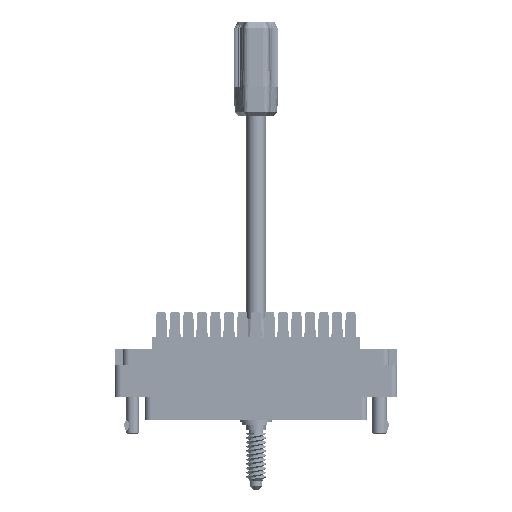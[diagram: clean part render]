
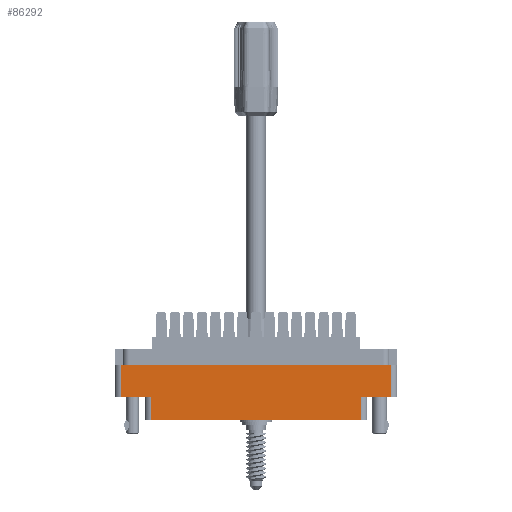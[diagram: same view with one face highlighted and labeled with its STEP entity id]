
A CAD part, front view. The second image highlights one B-rep face of the part: STEP entity #86292.
In plain terms, the highlighted planar face has unit normal (0, -1, 0).
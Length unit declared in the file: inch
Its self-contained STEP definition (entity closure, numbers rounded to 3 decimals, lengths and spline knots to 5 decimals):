
#207 = DIRECTION ( 'NONE',  ( 0., 0., 1. ) ) ;
#509 = ORIENTED_EDGE ( 'NONE', *, *, #36326, .T. ) ;
#2668 = DIRECTION ( 'NONE',  ( 0., 0., -1. ) ) ;
#3588 = LINE ( 'NONE', #40459, #69373 ) ;
#4038 = CARTESIAN_POINT ( 'NONE',  ( 1.297, -0.617, -0.274 ) ) ;
#4626 = LINE ( 'NONE', #34796, #83171 ) ;
#4710 = VECTOR ( 'NONE', #207, 39.37008 ) ;
#4845 = ORIENTED_EDGE ( 'NONE', *, *, #82349, .F. ) ;
#5252 = AXIS2_PLACEMENT_3D ( 'NONE', #71530, #87282, #94464 ) ;
#6112 = VECTOR ( 'NONE', #2668, 39.37008 ) ;
#8392 = DIRECTION ( 'NONE',  ( 1., 0., 0. ) ) ;
#12660 = ORIENTED_EDGE ( 'NONE', *, *, #57165, .T. ) ;
#14099 = PLANE ( 'NONE',  #5252 ) ;
#14154 = CARTESIAN_POINT ( 'NONE',  ( 0., -0.617, -0.578 ) ) ;
#14768 = VECTOR ( 'NONE', #71853, 39.37008 ) ;
#15088 = VECTOR ( 'NONE', #8392, 39.37008 ) ;
#15172 = EDGE_CURVE ( 'NONE', #60997, #40685, #4626, .T. ) ;
#16818 = ORIENTED_EDGE ( 'NONE', *, *, #30113, .T. ) ;
#22780 = VECTOR ( 'NONE', #74301, 39.37008 ) ;
#24410 = VERTEX_POINT ( 'NONE', #26943 ) ;
#26943 = CARTESIAN_POINT ( 'NONE',  ( 1.006, -0.617, -0.798 ) ) ;
#27652 = ORIENTED_EDGE ( 'NONE', *, *, #47729, .T. ) ;
#30113 = EDGE_CURVE ( 'NONE', #38169, #68191, #42983, .T. ) ;
#34769 = DIRECTION ( 'NONE',  ( -1., 0., 0. ) ) ;
#34796 = CARTESIAN_POINT ( 'NONE',  ( 0., -0.617, -0.274 ) ) ;
#36326 = EDGE_CURVE ( 'NONE', #81935, #24410, #3588, .T. ) ;
#38169 = VERTEX_POINT ( 'NONE', #83240 ) ;
#40459 = CARTESIAN_POINT ( 'NONE',  ( -1.359, -0.617, -0.798 ) ) ;
#40685 = VERTEX_POINT ( 'NONE', #4038 ) ;
#41538 = ORIENTED_EDGE ( 'NONE', *, *, #15172, .F. ) ;
#42349 = FACE_OUTER_BOUND ( 'NONE', #79198, .T. ) ;
#42983 = LINE ( 'NONE', #94177, #15088 ) ;
#44642 = CARTESIAN_POINT ( 'NONE',  ( 1.297, -0.617, -0.798 ) ) ;
#46209 = DIRECTION ( 'NONE',  ( 1., 0., 0. ) ) ;
#47729 = EDGE_CURVE ( 'NONE', #68191, #81935, #87598, .T. ) ;
#50055 = LINE ( 'NONE', #14154, #91768 ) ;
#51841 = LINE ( 'NONE', #44642, #22780 ) ;
#52334 = LINE ( 'NONE', #65763, #4710 ) ;
#54744 = EDGE_CURVE ( 'NONE', #60089, #40685, #51841, .T. ) ;
#55280 = VERTEX_POINT ( 'NONE', #68440 ) ;
#57070 = CARTESIAN_POINT ( 'NONE',  ( -1.297, -0.617, -0.274 ) ) ;
#57165 = EDGE_CURVE ( 'NONE', #24410, #55280, #52334, .T. ) ;
#60089 = VERTEX_POINT ( 'NONE', #87663 ) ;
#60997 = VERTEX_POINT ( 'NONE', #57070 ) ;
#65566 = CARTESIAN_POINT ( 'NONE',  ( -1.006, -0.617, -0.578 ) ) ;
#65605 = CARTESIAN_POINT ( 'NONE',  ( -1.006, -0.617, -0.798 ) ) ;
#65763 = CARTESIAN_POINT ( 'NONE',  ( 1.006, -0.617, -0.578 ) ) ;
#68191 = VERTEX_POINT ( 'NONE', #65566 ) ;
#68440 = CARTESIAN_POINT ( 'NONE',  ( 1.006, -0.617, -0.578 ) ) ;
#68733 = ORIENTED_EDGE ( 'NONE', *, *, #54744, .T. ) ;
#69373 = VECTOR ( 'NONE', #46209, 39.37008 ) ;
#71530 = CARTESIAN_POINT ( 'NONE',  ( -1.359, -0.617, -0.798 ) ) ;
#71853 = DIRECTION ( 'NONE',  ( 0., 0., -1. ) ) ;
#72638 = CARTESIAN_POINT ( 'NONE',  ( -1.006, -0.617, -0.798 ) ) ;
#74301 = DIRECTION ( 'NONE',  ( 0., 0., 1. ) ) ;
#77956 = EDGE_CURVE ( 'NONE', #60997, #38169, #83521, .T. ) ;
#79198 = EDGE_LOOP ( 'NONE', ( #16818, #27652, #509, #12660, #4845, #68733, #41538, #91367 ) ) ;
#79234 = DIRECTION ( 'NONE',  ( 1., 0., 0. ) ) ;
#81935 = VERTEX_POINT ( 'NONE', #72638 ) ;
#82349 = EDGE_CURVE ( 'NONE', #60089, #55280, #50055, .T. ) ;
#83171 = VECTOR ( 'NONE', #79234, 39.37008 ) ;
#83240 = CARTESIAN_POINT ( 'NONE',  ( -1.297, -0.617, -0.578 ) ) ;
#83521 = LINE ( 'NONE', #91616, #6112 ) ;
#86292 = ADVANCED_FACE ( 'NONE', ( #42349 ), #14099, .T. ) ;
#87282 = DIRECTION ( 'NONE',  ( 0., -1., 0. ) ) ;
#87598 = LINE ( 'NONE', #65605, #14768 ) ;
#87663 = CARTESIAN_POINT ( 'NONE',  ( 1.297, -0.617, -0.578 ) ) ;
#91367 = ORIENTED_EDGE ( 'NONE', *, *, #77956, .T. ) ;
#91616 = CARTESIAN_POINT ( 'NONE',  ( -1.297, -0.617, -0.798 ) ) ;
#91768 = VECTOR ( 'NONE', #34769, 39.37008 ) ;
#94177 = CARTESIAN_POINT ( 'NONE',  ( 0., -0.617, -0.578 ) ) ;
#94464 = DIRECTION ( 'NONE',  ( 0., 0., -1. ) ) ;
